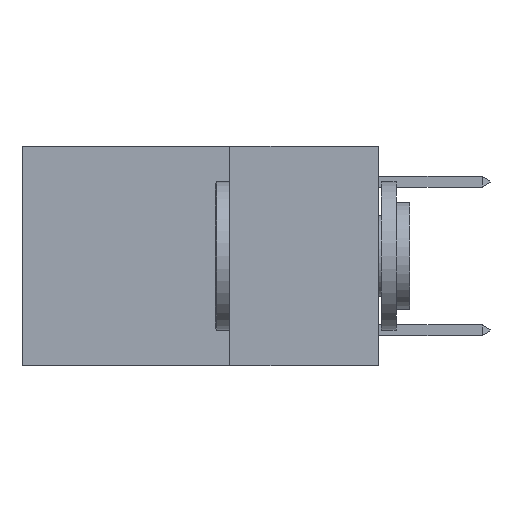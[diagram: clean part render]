
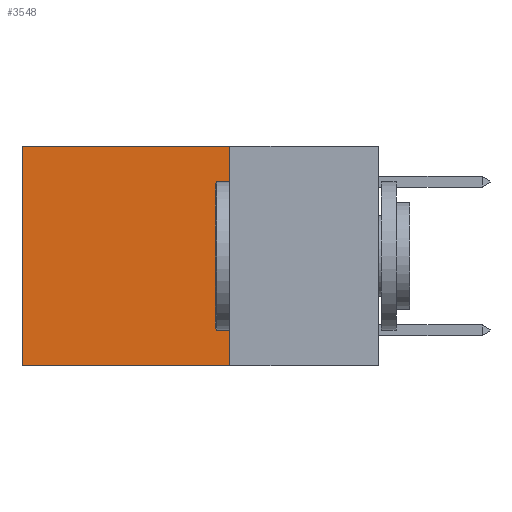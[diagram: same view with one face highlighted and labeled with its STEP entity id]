
A CAD part, left-side view. The second image highlights one B-rep face of the part: STEP entity #3548.
In plain terms, the highlighted planar face has unit normal (-1, 0, 0).
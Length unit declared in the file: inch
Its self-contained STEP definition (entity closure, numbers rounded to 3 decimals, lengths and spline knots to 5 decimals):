
#66 = DIRECTION ( 'NONE',  ( 0., 1., 0. ) ) ;
#727 = CARTESIAN_POINT ( 'NONE',  ( 0.2625, 0.25, 0. ) ) ;
#1047 = VECTOR ( 'NONE', #15279, 39.37008 ) ;
#1369 = CARTESIAN_POINT ( 'NONE',  ( 0.2625, 0.25, -0.37 ) ) ;
#2453 = VECTOR ( 'NONE', #12844, 39.37008 ) ;
#2595 = DIRECTION ( 'NONE',  ( 1., 0., 0. ) ) ;
#2674 = CARTESIAN_POINT ( 'NONE',  ( 0.2625, 0.6, 0. ) ) ;
#2926 = AXIS2_PLACEMENT_3D ( 'NONE', #18049, #2595, #19386 ) ;
#2927 = LINE ( 'NONE', #727, #15380 ) ;
#3548 = ADVANCED_FACE ( 'NONE', ( #12850 ), #12748, .F. ) ;
#4798 = CARTESIAN_POINT ( 'NONE',  ( 0.2625, 0.25, -0.37 ) ) ;
#4873 = CARTESIAN_POINT ( 'NONE',  ( 0.2625, 0.25, 0. ) ) ;
#6179 = EDGE_CURVE ( 'NONE', #10790, #21790, #20136, .T. ) ;
#6209 = ORIENTED_EDGE ( 'NONE', *, *, #9845, .T. ) ;
#6645 = LINE ( 'NONE', #13443, #15697 ) ;
#6940 = EDGE_CURVE ( 'NONE', #14899, #19669, #2927, .T. ) ;
#7492 = DIRECTION ( 'NONE',  ( 0., 0., -1. ) ) ;
#9845 = EDGE_CURVE ( 'NONE', #14899, #10790, #6645, .T. ) ;
#10184 = CARTESIAN_POINT ( 'NONE',  ( 0.2625, 0.6, 0. ) ) ;
#10790 = VERTEX_POINT ( 'NONE', #2674 ) ;
#10796 = ORIENTED_EDGE ( 'NONE', *, *, #6940, .F. ) ;
#10952 = ORIENTED_EDGE ( 'NONE', *, *, #14287, .F. ) ;
#11503 = LINE ( 'NONE', #1369, #2453 ) ;
#12748 = PLANE ( 'NONE',  #2926 ) ;
#12844 = DIRECTION ( 'NONE',  ( 0., 1., 0. ) ) ;
#12850 = FACE_OUTER_BOUND ( 'NONE', #13249, .T. ) ;
#13249 = EDGE_LOOP ( 'NONE', ( #16311, #10952, #10796, #6209 ) ) ;
#13443 = CARTESIAN_POINT ( 'NONE',  ( 0.2625, 0.25, 0. ) ) ;
#14287 = EDGE_CURVE ( 'NONE', #19669, #21790, #11503, .T. ) ;
#14899 = VERTEX_POINT ( 'NONE', #4873 ) ;
#15279 = DIRECTION ( 'NONE',  ( 0., 0., -1. ) ) ;
#15380 = VECTOR ( 'NONE', #7492, 39.37008 ) ;
#15697 = VECTOR ( 'NONE', #66, 39.37008 ) ;
#16311 = ORIENTED_EDGE ( 'NONE', *, *, #6179, .T. ) ;
#18049 = CARTESIAN_POINT ( 'NONE',  ( 0.2625, 0.25, 0. ) ) ;
#19386 = DIRECTION ( 'NONE',  ( 0., 0., -1. ) ) ;
#19669 = VERTEX_POINT ( 'NONE', #4798 ) ;
#20136 = LINE ( 'NONE', #10184, #1047 ) ;
#20516 = CARTESIAN_POINT ( 'NONE',  ( 0.2625, 0.6, -0.37 ) ) ;
#21790 = VERTEX_POINT ( 'NONE', #20516 ) ;
